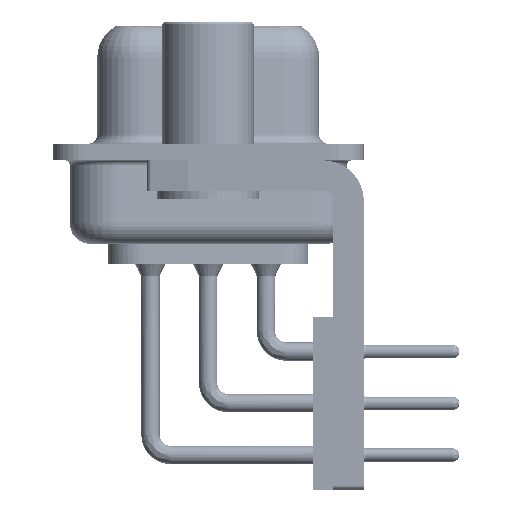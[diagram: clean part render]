
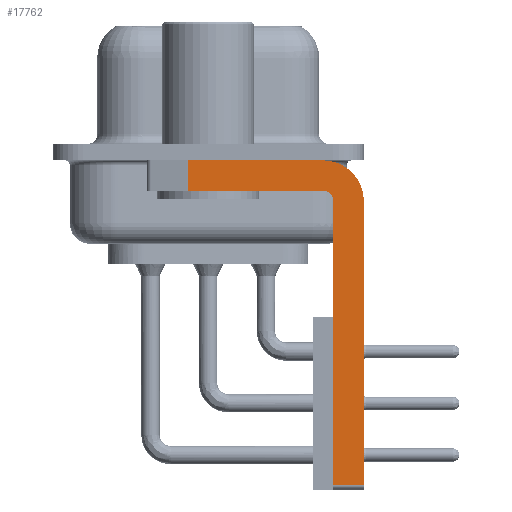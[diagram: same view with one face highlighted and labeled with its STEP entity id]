
A CAD part, left-side view. The second image highlights one B-rep face of the part: STEP entity #17762.
In plain terms, the highlighted planar face has unit normal (-1, 0, 0).
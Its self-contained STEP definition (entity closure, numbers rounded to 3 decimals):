
#1137 = CARTESIAN_POINT ( 'NONE',  ( -2.9, -5.65, -1.9 ) ) ;
#1591 = DIRECTION ( 'NONE',  ( -1., 0., 0. ) ) ;
#1729 = CARTESIAN_POINT ( 'NONE',  ( -2.9, -7.65, -16.35 ) ) ;
#2147 = EDGE_CURVE ( 'NONE', #18755, #32890, #31909, .T. ) ;
#2265 = DIRECTION ( 'NONE',  ( 0., 0., -1. ) ) ;
#2722 = ORIENTED_EDGE ( 'NONE', *, *, #11657, .T. ) ;
#2964 = ORIENTED_EDGE ( 'NONE', *, *, #21944, .F. ) ;
#3125 = LINE ( 'NONE', #1137, #32452 ) ;
#3732 = CIRCLE ( 'NONE', #10000, 0.5 ) ;
#4927 = DIRECTION ( 'NONE',  ( 0., 0., -1. ) ) ;
#4957 = VECTOR ( 'NONE', #9077, 1000. ) ;
#5238 = VECTOR ( 'NONE', #32576, 1000. ) ;
#7806 = VECTOR ( 'NONE', #4927, 1000. ) ;
#7986 = ORIENTED_EDGE ( 'NONE', *, *, #21234, .F. ) ;
#8059 = CARTESIAN_POINT ( 'NONE',  ( -2.9, 0.978, -1.9 ) ) ;
#8090 = EDGE_CURVE ( 'NONE', #9751, #27248, #29638, .T. ) ;
#9077 = DIRECTION ( 'NONE',  ( 0., -1., 0. ) ) ;
#9130 = ORIENTED_EDGE ( 'NONE', *, *, #13764, .F. ) ;
#9675 = DIRECTION ( 'NONE',  ( 0., 0., 1. ) ) ;
#9751 = VERTEX_POINT ( 'NONE', #20942 ) ;
#10000 = AXIS2_PLACEMENT_3D ( 'NONE', #19746, #1591, #22781 ) ;
#10141 = CIRCLE ( 'NONE', #30768, 2. ) ;
#10284 = DIRECTION ( 'NONE',  ( 0., 1., 0. ) ) ;
#11423 = CARTESIAN_POINT ( 'NONE',  ( -2.9, -6.15, -2.4 ) ) ;
#11487 = CARTESIAN_POINT ( 'NONE',  ( -2.9, -7.65, -2.4 ) ) ;
#11657 = EDGE_CURVE ( 'NONE', #9751, #31919, #14701, .T. ) ;
#11790 = EDGE_CURVE ( 'NONE', #27248, #13528, #3732, .T. ) ;
#12455 = ORIENTED_EDGE ( 'NONE', *, *, #2147, .T. ) ;
#13341 = CARTESIAN_POINT ( 'NONE',  ( -2.9, -5.65, -2.4 ) ) ;
#13528 = VERTEX_POINT ( 'NONE', #26761 ) ;
#13764 = EDGE_CURVE ( 'NONE', #13528, #32890, #3125, .T. ) ;
#14154 = VERTEX_POINT ( 'NONE', #26974 ) ;
#14382 = PLANE ( 'NONE',  #24112 ) ;
#14701 = LINE ( 'NONE', #34008, #36907 ) ;
#15251 = ORIENTED_EDGE ( 'NONE', *, *, #17169, .F. ) ;
#16392 = DIRECTION ( 'NONE',  ( 0., 0., -1. ) ) ;
#17169 = EDGE_CURVE ( 'NONE', #17811, #31919, #37446, .T. ) ;
#17403 = CARTESIAN_POINT ( 'NONE',  ( -2.9, -5.65, -2.4 ) ) ;
#17762 = ADVANCED_FACE ( 'NONE', ( #23173 ), #14382, .F. ) ;
#17811 = VERTEX_POINT ( 'NONE', #29608 ) ;
#18755 = VERTEX_POINT ( 'NONE', #37299 ) ;
#19746 = CARTESIAN_POINT ( 'NONE',  ( -2.9, -5.65, -2.4 ) ) ;
#20433 = DIRECTION ( 'NONE',  ( 1., 0., 0. ) ) ;
#20942 = CARTESIAN_POINT ( 'NONE',  ( -2.9, -6.15, -16.35 ) ) ;
#21069 = LINE ( 'NONE', #27127, #4957 ) ;
#21234 = EDGE_CURVE ( 'NONE', #14154, #17811, #10141, .T. ) ;
#21658 = VECTOR ( 'NONE', #9675, 1000. ) ;
#21723 = CARTESIAN_POINT ( 'NONE',  ( -2.9, -6.15, -16.6 ) ) ;
#21944 = EDGE_CURVE ( 'NONE', #18755, #14154, #21069, .T. ) ;
#22781 = DIRECTION ( 'NONE',  ( 0., 0., 1. ) ) ;
#23173 = FACE_OUTER_BOUND ( 'NONE', #26457, .T. ) ;
#24112 = AXIS2_PLACEMENT_3D ( 'NONE', #17403, #20433, #2265 ) ;
#26457 = EDGE_LOOP ( 'NONE', ( #2964, #12455, #9130, #26687, #37765, #2722, #15251, #7986 ) ) ;
#26687 = ORIENTED_EDGE ( 'NONE', *, *, #11790, .F. ) ;
#26761 = CARTESIAN_POINT ( 'NONE',  ( -2.9, -5.65, -1.9 ) ) ;
#26974 = CARTESIAN_POINT ( 'NONE',  ( -2.9, -5.65, -0.4 ) ) ;
#27127 = CARTESIAN_POINT ( 'NONE',  ( -2.9, 3., -0.4 ) ) ;
#27248 = VERTEX_POINT ( 'NONE', #11423 ) ;
#27942 = CARTESIAN_POINT ( 'NONE',  ( -2.9, 0.978, -1.9 ) ) ;
#29608 = CARTESIAN_POINT ( 'NONE',  ( -2.9, -7.65, -2.4 ) ) ;
#29638 = LINE ( 'NONE', #21723, #21658 ) ;
#30768 = AXIS2_PLACEMENT_3D ( 'NONE', #13341, #34465, #16392 ) ;
#30937 = DIRECTION ( 'NONE',  ( 0., -1., 0. ) ) ;
#31909 = LINE ( 'NONE', #8059, #7806 ) ;
#31919 = VERTEX_POINT ( 'NONE', #1729 ) ;
#32452 = VECTOR ( 'NONE', #10284, 1000. ) ;
#32576 = DIRECTION ( 'NONE',  ( 0., 0., -1. ) ) ;
#32890 = VERTEX_POINT ( 'NONE', #27942 ) ;
#34008 = CARTESIAN_POINT ( 'NONE',  ( -2.9, -5.65, -16.35 ) ) ;
#34465 = DIRECTION ( 'NONE',  ( 1., 0., 0. ) ) ;
#36907 = VECTOR ( 'NONE', #30937, 1000. ) ;
#37299 = CARTESIAN_POINT ( 'NONE',  ( -2.9, 0.978, -0.4 ) ) ;
#37446 = LINE ( 'NONE', #11487, #5238 ) ;
#37765 = ORIENTED_EDGE ( 'NONE', *, *, #8090, .F. ) ;
